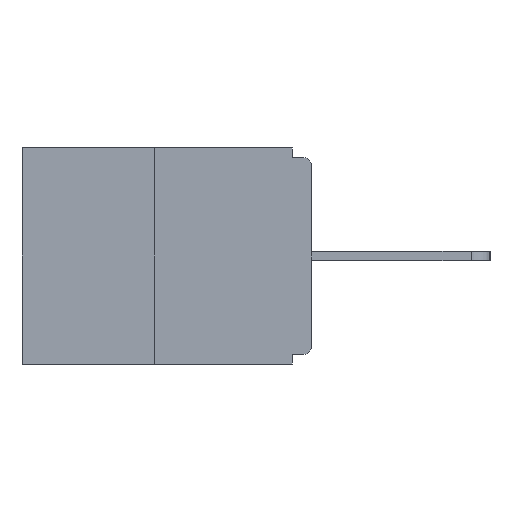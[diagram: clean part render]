
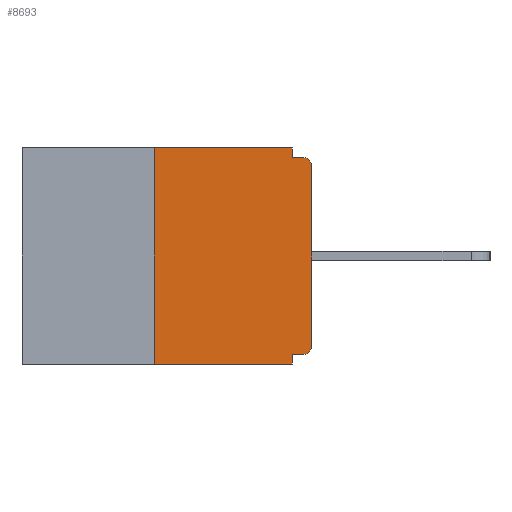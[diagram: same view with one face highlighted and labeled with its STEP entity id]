
A CAD part, left-side view. The second image highlights one B-rep face of the part: STEP entity #8693.
In plain terms, the highlighted planar face has unit normal (-1, 0, 0).
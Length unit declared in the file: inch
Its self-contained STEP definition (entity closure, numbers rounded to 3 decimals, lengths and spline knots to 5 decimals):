
#244 = DIRECTION ( 'NONE',  ( 0., -1., 0. ) ) ;
#386 = LINE ( 'NONE', #12631, #8308 ) ;
#487 = VERTEX_POINT ( 'NONE', #1983 ) ;
#985 = VERTEX_POINT ( 'NONE', #2351 ) ;
#1070 = VERTEX_POINT ( 'NONE', #15713 ) ;
#1184 = EDGE_CURVE ( 'NONE', #1070, #7528, #11909, .T. ) ;
#1474 = PLANE ( 'NONE',  #13923 ) ;
#1617 = CARTESIAN_POINT ( 'NONE',  ( 0., 0.46, 0. ) ) ;
#1962 = CARTESIAN_POINT ( 'NONE',  ( 0., 0.031, 0. ) ) ;
#1983 = CARTESIAN_POINT ( 'NONE',  ( 0., 0.031, -0.343 ) ) ;
#2327 = ORIENTED_EDGE ( 'NONE', *, *, #19200, .F. ) ;
#2351 = CARTESIAN_POINT ( 'NONE',  ( 0., 0.25, 0. ) ) ;
#2704 = CARTESIAN_POINT ( 'NONE',  ( 0., 0.031, -0.328 ) ) ;
#3084 = ORIENTED_EDGE ( 'NONE', *, *, #9828, .T. ) ;
#3271 = ORIENTED_EDGE ( 'NONE', *, *, #1184, .T. ) ;
#3523 = CARTESIAN_POINT ( 'NONE',  ( 0., 0.25, -0.343 ) ) ;
#3526 = DIRECTION ( 'NONE',  ( 0., 0., -1. ) ) ;
#3541 = ORIENTED_EDGE ( 'NONE', *, *, #10146, .F. ) ;
#3719 = CARTESIAN_POINT ( 'NONE',  ( 0., 0.031, -0.343 ) ) ;
#3874 = CIRCLE ( 'NONE', #18504, 0.015 ) ;
#4432 = CARTESIAN_POINT ( 'NONE',  ( 0., 0.015, -0.03 ) ) ;
#4542 = VERTEX_POINT ( 'NONE', #1962 ) ;
#4701 = LINE ( 'NONE', #10789, #16963 ) ;
#4849 = VERTEX_POINT ( 'NONE', #17350 ) ;
#5026 = VERTEX_POINT ( 'NONE', #2704 ) ;
#5523 = DIRECTION ( 'NONE',  ( 0., 0., -1. ) ) ;
#5900 = DIRECTION ( 'NONE',  ( -1., 0., 0. ) ) ;
#6408 = ORIENTED_EDGE ( 'NONE', *, *, #14286, .T. ) ;
#6666 = VECTOR ( 'NONE', #3526, 39.37008 ) ;
#7528 = VERTEX_POINT ( 'NONE', #13652 ) ;
#7536 = CARTESIAN_POINT ( 'NONE',  ( 0., 0.46, 0. ) ) ;
#7797 = DIRECTION ( 'NONE',  ( 0., 0., -1. ) ) ;
#8131 = DIRECTION ( 'NONE',  ( 0., 0., 1. ) ) ;
#8308 = VECTOR ( 'NONE', #8131, 39.37008 ) ;
#8597 = LINE ( 'NONE', #10849, #19358 ) ;
#8693 = ADVANCED_FACE ( 'NONE', ( #15142 ), #1474, .F. ) ;
#9095 = LINE ( 'NONE', #1617, #12216 ) ;
#9321 = VECTOR ( 'NONE', #17547, 39.37008 ) ;
#9828 = EDGE_CURVE ( 'NONE', #10837, #487, #8597, .T. ) ;
#10146 = EDGE_CURVE ( 'NONE', #13653, #7528, #12940, .T. ) ;
#10239 = DIRECTION ( 'NONE',  ( 0., -1., 0. ) ) ;
#10451 = VECTOR ( 'NONE', #12494, 39.37008 ) ;
#10513 = DIRECTION ( 'NONE',  ( -1., 0., 0. ) ) ;
#10751 = VERTEX_POINT ( 'NONE', #19569 ) ;
#10754 = DIRECTION ( 'NONE',  ( 0., -1., 0. ) ) ;
#10789 = CARTESIAN_POINT ( 'NONE',  ( 0., 0.25, 0. ) ) ;
#10837 = VERTEX_POINT ( 'NONE', #3523 ) ;
#10849 = CARTESIAN_POINT ( 'NONE',  ( 0., 0.46, -0.343 ) ) ;
#11233 = ORIENTED_EDGE ( 'NONE', *, *, #15515, .F. ) ;
#11534 = CARTESIAN_POINT ( 'NONE',  ( 0., 0., -0.015 ) ) ;
#11653 = EDGE_CURVE ( 'NONE', #5026, #487, #18765, .T. ) ;
#11909 = CIRCLE ( 'NONE', #17305, 0.015 ) ;
#12216 = VECTOR ( 'NONE', #244, 39.37008 ) ;
#12374 = EDGE_CURVE ( 'NONE', #10751, #1070, #386, .T. ) ;
#12494 = DIRECTION ( 'NONE',  ( 0., 0., -1. ) ) ;
#12631 = CARTESIAN_POINT ( 'NONE',  ( 0., 0., 0. ) ) ;
#12704 = VECTOR ( 'NONE', #10239, 39.37008 ) ;
#12940 = LINE ( 'NONE', #11534, #12704 ) ;
#13059 = EDGE_LOOP ( 'NONE', ( #13291, #11233, #3084, #16102, #16871, #6408, #13638, #3271, #3541, #2327 ) ) ;
#13291 = ORIENTED_EDGE ( 'NONE', *, *, #16790, .F. ) ;
#13638 = ORIENTED_EDGE ( 'NONE', *, *, #12374, .T. ) ;
#13652 = CARTESIAN_POINT ( 'NONE',  ( 0., 0.015, -0.015 ) ) ;
#13653 = VERTEX_POINT ( 'NONE', #14516 ) ;
#13752 = DIRECTION ( 'NONE',  ( 1., 0., 0. ) ) ;
#13923 = AXIS2_PLACEMENT_3D ( 'NONE', #7536, #13752, #17123 ) ;
#14078 = LINE ( 'NONE', #14174, #9321 ) ;
#14174 = CARTESIAN_POINT ( 'NONE',  ( 0., 0., -0.328 ) ) ;
#14286 = EDGE_CURVE ( 'NONE', #4849, #10751, #3874, .T. ) ;
#14516 = CARTESIAN_POINT ( 'NONE',  ( 0., 0.031, -0.015 ) ) ;
#15142 = FACE_OUTER_BOUND ( 'NONE', #13059, .T. ) ;
#15515 = EDGE_CURVE ( 'NONE', #10837, #985, #4701, .T. ) ;
#15643 = EDGE_CURVE ( 'NONE', #4849, #5026, #14078, .T. ) ;
#15713 = CARTESIAN_POINT ( 'NONE',  ( 0., 0., -0.03 ) ) ;
#16102 = ORIENTED_EDGE ( 'NONE', *, *, #11653, .F. ) ;
#16790 = EDGE_CURVE ( 'NONE', #985, #4542, #9095, .T. ) ;
#16871 = ORIENTED_EDGE ( 'NONE', *, *, #15643, .F. ) ;
#16872 = DIRECTION ( 'NONE',  ( 0., 0., 1. ) ) ;
#16963 = VECTOR ( 'NONE', #16872, 39.37008 ) ;
#17123 = DIRECTION ( 'NONE',  ( 0., 0., -1. ) ) ;
#17166 = CARTESIAN_POINT ( 'NONE',  ( 0., 0.031, 0. ) ) ;
#17258 = LINE ( 'NONE', #17166, #10451 ) ;
#17305 = AXIS2_PLACEMENT_3D ( 'NONE', #4432, #10513, #5523 ) ;
#17350 = CARTESIAN_POINT ( 'NONE',  ( 0., 0.015, -0.328 ) ) ;
#17547 = DIRECTION ( 'NONE',  ( 0., 1., 0. ) ) ;
#18504 = AXIS2_PLACEMENT_3D ( 'NONE', #19559, #5900, #7797 ) ;
#18765 = LINE ( 'NONE', #3719, #6666 ) ;
#19200 = EDGE_CURVE ( 'NONE', #4542, #13653, #17258, .T. ) ;
#19358 = VECTOR ( 'NONE', #10754, 39.37008 ) ;
#19559 = CARTESIAN_POINT ( 'NONE',  ( 0., 0.015, -0.313 ) ) ;
#19569 = CARTESIAN_POINT ( 'NONE',  ( 0., 0., -0.313 ) ) ;
